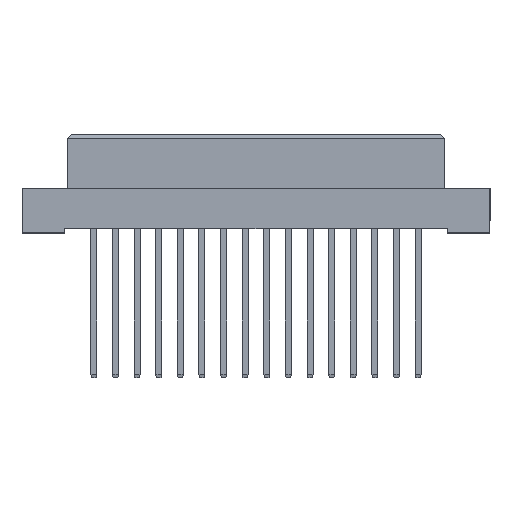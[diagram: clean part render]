
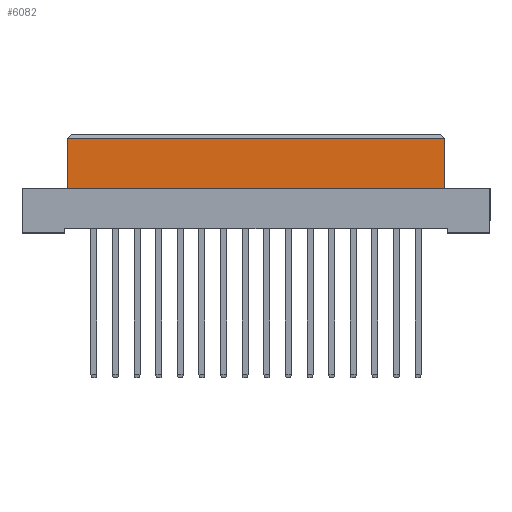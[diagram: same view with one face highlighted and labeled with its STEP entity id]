
A CAD part, top view. The second image highlights one B-rep face of the part: STEP entity #6082.
In plain terms, the highlighted planar face has unit normal (0, 0, 1).
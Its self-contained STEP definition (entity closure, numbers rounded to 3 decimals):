
#1234 = ORIENTED_EDGE ( 'NONE', *, *, #6496, .T. ) ;
#1828 = AXIS2_PLACEMENT_3D ( 'NONE', #17725, #6493, #15995 ) ;
#2698 = DIRECTION ( 'NONE',  ( 0., 1., 0. ) ) ;
#3218 = CARTESIAN_POINT ( 'NONE',  ( 22.2, -6.4, 4.25 ) ) ;
#3895 = CARTESIAN_POINT ( 'NONE',  ( 22.2, -6.4, 4.25 ) ) ;
#4057 = VERTEX_POINT ( 'NONE', #17449 ) ;
#4830 = LINE ( 'NONE', #3218, #15562 ) ;
#5561 = CARTESIAN_POINT ( 'NONE',  ( -22.2, -6.4, 4.25 ) ) ;
#6082 = ADVANCED_FACE ( 'NONE', ( #19445 ), #9408, .T. ) ;
#6140 = ORIENTED_EDGE ( 'NONE', *, *, #10454, .T. ) ;
#6162 = DIRECTION ( 'NONE',  ( -1., 0., 0. ) ) ;
#6493 = DIRECTION ( 'NONE',  ( 0., 0., 1. ) ) ;
#6496 = EDGE_CURVE ( 'NONE', #17075, #17086, #11100, .T. ) ;
#6915 = EDGE_CURVE ( 'NONE', #10155, #17086, #19186, .T. ) ;
#7617 = ORIENTED_EDGE ( 'NONE', *, *, #16145, .T. ) ;
#9408 = PLANE ( 'NONE',  #1828 ) ;
#10155 = VERTEX_POINT ( 'NONE', #5561 ) ;
#10238 = CARTESIAN_POINT ( 'NONE',  ( -22.2, -0.5, 4.25 ) ) ;
#10441 = LINE ( 'NONE', #3895, #11666 ) ;
#10454 = EDGE_CURVE ( 'NONE', #10155, #4057, #10441, .T. ) ;
#10466 = EDGE_LOOP ( 'NONE', ( #7617, #1234, #16575, #6140 ) ) ;
#11100 = LINE ( 'NONE', #21242, #14293 ) ;
#11666 = VECTOR ( 'NONE', #13672, 1000. ) ;
#12947 = CARTESIAN_POINT ( 'NONE',  ( 22.2, -0.5, 4.25 ) ) ;
#13672 = DIRECTION ( 'NONE',  ( 1., 0., 0. ) ) ;
#14293 = VECTOR ( 'NONE', #6162, 1000. ) ;
#14728 = DIRECTION ( 'NONE',  ( 0., 1., 0. ) ) ;
#15562 = VECTOR ( 'NONE', #14728, 1000. ) ;
#15995 = DIRECTION ( 'NONE',  ( 1., 0., 0. ) ) ;
#16145 = EDGE_CURVE ( 'NONE', #4057, #17075, #4830, .T. ) ;
#16575 = ORIENTED_EDGE ( 'NONE', *, *, #6915, .F. ) ;
#16685 = VECTOR ( 'NONE', #2698, 1000. ) ;
#17075 = VERTEX_POINT ( 'NONE', #12947 ) ;
#17086 = VERTEX_POINT ( 'NONE', #10238 ) ;
#17449 = CARTESIAN_POINT ( 'NONE',  ( 22.2, -6.4, 4.25 ) ) ;
#17725 = CARTESIAN_POINT ( 'NONE',  ( 22.2, -6.4, 4.25 ) ) ;
#19186 = LINE ( 'NONE', #19295, #16685 ) ;
#19295 = CARTESIAN_POINT ( 'NONE',  ( -22.2, -6.4, 4.25 ) ) ;
#19445 = FACE_OUTER_BOUND ( 'NONE', #10466, .T. ) ;
#21242 = CARTESIAN_POINT ( 'NONE',  ( -22.2, -0.5, 4.25 ) ) ;
